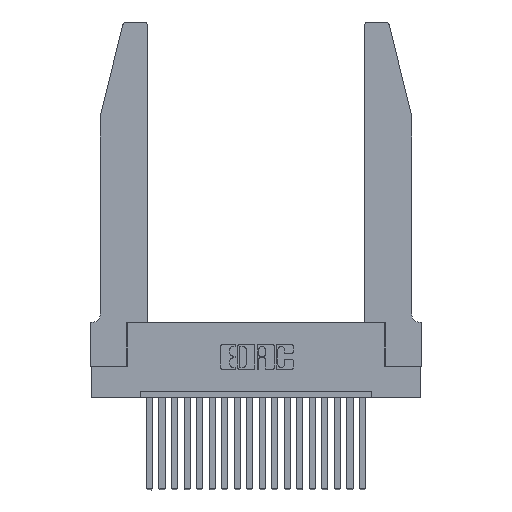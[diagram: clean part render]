
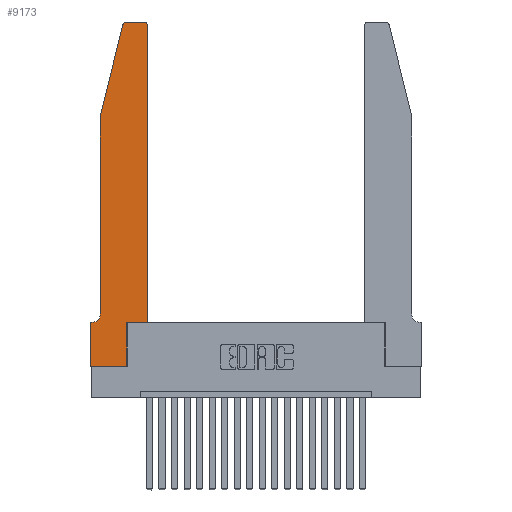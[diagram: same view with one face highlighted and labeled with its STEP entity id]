
A CAD part, top view. The second image highlights one B-rep face of the part: STEP entity #9173.
In plain terms, the highlighted planar face has unit normal (0, 0, 1).
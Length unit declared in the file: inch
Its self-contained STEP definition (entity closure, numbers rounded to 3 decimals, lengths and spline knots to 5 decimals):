
#276 = VERTEX_POINT ( 'NONE', #17920 ) ;
#367 = EDGE_CURVE ( 'NONE', #18900, #5737, #6683, .T. ) ;
#470 = CARTESIAN_POINT ( 'NONE',  ( 0., 0.35, 0.37 ) ) ;
#474 = CARTESIAN_POINT ( 'NONE',  ( 0.0755, 2., 0.37 ) ) ;
#629 = ORIENTED_EDGE ( 'NONE', *, *, #16393, .T. ) ;
#804 = CARTESIAN_POINT ( 'NONE',  ( 0.284, 2.72, 0.37 ) ) ;
#1341 = CARTESIAN_POINT ( 'NONE',  ( 0., 0.35, 0.37 ) ) ;
#1422 = VERTEX_POINT ( 'NONE', #15681 ) ;
#1963 = DIRECTION ( 'NONE',  ( 0., 1., 0. ) ) ;
#1997 = VERTEX_POINT ( 'NONE', #16521 ) ;
#2380 = ORIENTED_EDGE ( 'NONE', *, *, #7766, .T. ) ;
#2518 = DIRECTION ( 'NONE',  ( 1., 0., 0. ) ) ;
#2613 = LINE ( 'NONE', #474, #13183 ) ;
#2767 = VECTOR ( 'NONE', #1963, 39.37008 ) ;
#3095 = LINE ( 'NONE', #8594, #20072 ) ;
#3139 = CARTESIAN_POINT ( 'NONE',  ( 0.2865, 0., 0.37 ) ) ;
#3298 = ORIENTED_EDGE ( 'NONE', *, *, #17960, .T. ) ;
#3741 = CARTESIAN_POINT ( 'NONE',  ( 0.4205, 2.75, 0.37 ) ) ;
#3867 = VECTOR ( 'NONE', #13098, 39.37008 ) ;
#4355 = VERTEX_POINT ( 'NONE', #9360 ) ;
#4455 = VERTEX_POINT ( 'NONE', #3139 ) ;
#4566 = CARTESIAN_POINT ( 'NONE',  ( 0.0755, 2., 0.37 ) ) ;
#4745 = CARTESIAN_POINT ( 'NONE',  ( 0.25487, 2.72718, 0.37 ) ) ;
#4773 = VECTOR ( 'NONE', #19649, 39.37008 ) ;
#4788 = AXIS2_PLACEMENT_3D ( 'NONE', #14901, #16583, #8051 ) ;
#5555 = ORIENTED_EDGE ( 'NONE', *, *, #17258, .T. ) ;
#5737 = VERTEX_POINT ( 'NONE', #470 ) ;
#6047 = ORIENTED_EDGE ( 'NONE', *, *, #11536, .T. ) ;
#6191 = VECTOR ( 'NONE', #14361, 39.37008 ) ;
#6246 = DIRECTION ( 'NONE',  ( 0., 0., 1. ) ) ;
#6342 = CARTESIAN_POINT ( 'NONE',  ( 0.4505, 0.35, 0.37 ) ) ;
#6538 = DIRECTION ( 'NONE',  ( 1., 0., 0. ) ) ;
#6541 = VERTEX_POINT ( 'NONE', #4745 ) ;
#6654 = CARTESIAN_POINT ( 'NONE',  ( 0.2865, 0.35, 0.37 ) ) ;
#6683 = LINE ( 'NONE', #15209, #6191 ) ;
#6728 = CARTESIAN_POINT ( 'NONE',  ( 0.4505, 0.35, 0.37 ) ) ;
#7055 = DIRECTION ( 'NONE',  ( -1., 0., 0. ) ) ;
#7310 = ORIENTED_EDGE ( 'NONE', *, *, #21116, .T. ) ;
#7766 = EDGE_CURVE ( 'NONE', #19684, #18900, #10150, .T. ) ;
#7827 = PLANE ( 'NONE',  #13759 ) ;
#7865 = CARTESIAN_POINT ( 'NONE',  ( 0.4505, 2.72, 0.37 ) ) ;
#8051 = DIRECTION ( 'NONE',  ( 1., 0., 0. ) ) ;
#8155 = LINE ( 'NONE', #6342, #4773 ) ;
#8370 = CIRCLE ( 'NONE', #4788, 0.03 ) ;
#8379 = ORIENTED_EDGE ( 'NONE', *, *, #8538, .T. ) ;
#8538 = EDGE_CURVE ( 'NONE', #5737, #1997, #10610, .T. ) ;
#8594 = CARTESIAN_POINT ( 'NONE',  ( 0.2605, 2.75, 0.37 ) ) ;
#8809 = VECTOR ( 'NONE', #17312, 39.37008 ) ;
#9173 = ADVANCED_FACE ( 'NONE', ( #19567 ), #7827, .T. ) ;
#9360 = CARTESIAN_POINT ( 'NONE',  ( 0.4505, 0.35, 0.37 ) ) ;
#10059 = AXIS2_PLACEMENT_3D ( 'NONE', #804, #12324, #2518 ) ;
#10150 = CIRCLE ( 'NONE', #18430, 0.07 ) ;
#10610 = LINE ( 'NONE', #10720, #8809 ) ;
#10720 = CARTESIAN_POINT ( 'NONE',  ( 0., 0., 0.37 ) ) ;
#10819 = EDGE_CURVE ( 'NONE', #4455, #20757, #11882, .T. ) ;
#11406 = CARTESIAN_POINT ( 'NONE',  ( 0., 0., 0.37 ) ) ;
#11536 = EDGE_CURVE ( 'NONE', #13530, #1422, #3095, .T. ) ;
#11608 = ORIENTED_EDGE ( 'NONE', *, *, #367, .T. ) ;
#11882 = LINE ( 'NONE', #6654, #3867 ) ;
#12091 = CARTESIAN_POINT ( 'NONE',  ( 0.2865, 0.35, 0.37 ) ) ;
#12164 = LINE ( 'NONE', #4566, #18604 ) ;
#12324 = DIRECTION ( 'NONE',  ( 0., 0., 1. ) ) ;
#12583 = DIRECTION ( 'NONE',  ( -0.239, -0.971, 0. ) ) ;
#12602 = ORIENTED_EDGE ( 'NONE', *, *, #18326, .T. ) ;
#13098 = DIRECTION ( 'NONE',  ( 0., 1., 0. ) ) ;
#13183 = VECTOR ( 'NONE', #12583, 39.37008 ) ;
#13507 = ORIENTED_EDGE ( 'NONE', *, *, #20832, .T. ) ;
#13530 = VERTEX_POINT ( 'NONE', #3741 ) ;
#13759 = AXIS2_PLACEMENT_3D ( 'NONE', #1341, #6246, #19400 ) ;
#13806 = EDGE_LOOP ( 'NONE', ( #6047, #3298, #13507, #629, #2380, #11608, #8379, #12602, #14019, #13824, #5555, #7310 ) ) ;
#13824 = ORIENTED_EDGE ( 'NONE', *, *, #18267, .T. ) ;
#14019 = ORIENTED_EDGE ( 'NONE', *, *, #10819, .T. ) ;
#14361 = DIRECTION ( 'NONE',  ( -1., 0., 0. ) ) ;
#14372 = CARTESIAN_POINT ( 'NONE',  ( 0.0055, 0.35, 0.37 ) ) ;
#14901 = CARTESIAN_POINT ( 'NONE',  ( 0.4205, 2.72, 0.37 ) ) ;
#15209 = CARTESIAN_POINT ( 'NONE',  ( 0.0755, 0.35, 0.37 ) ) ;
#15681 = CARTESIAN_POINT ( 'NONE',  ( 0.284, 2.75, 0.37 ) ) ;
#16393 = EDGE_CURVE ( 'NONE', #276, #19684, #12164, .T. ) ;
#16521 = CARTESIAN_POINT ( 'NONE',  ( 0., 0., 0.37 ) ) ;
#16583 = DIRECTION ( 'NONE',  ( 0., 0., 1. ) ) ;
#16988 = DIRECTION ( 'NONE',  ( -1., 0., 0. ) ) ;
#17209 = LINE ( 'NONE', #6728, #2767 ) ;
#17258 = EDGE_CURVE ( 'NONE', #4355, #18194, #17209, .T. ) ;
#17312 = DIRECTION ( 'NONE',  ( 0., -1., 0. ) ) ;
#17692 = CIRCLE ( 'NONE', #10059, 0.03 ) ;
#17920 = CARTESIAN_POINT ( 'NONE',  ( 0.0755, 2., 0.37 ) ) ;
#17960 = EDGE_CURVE ( 'NONE', #1422, #6541, #17692, .T. ) ;
#18194 = VERTEX_POINT ( 'NONE', #7865 ) ;
#18267 = EDGE_CURVE ( 'NONE', #20757, #4355, #8155, .T. ) ;
#18326 = EDGE_CURVE ( 'NONE', #1997, #4455, #18704, .T. ) ;
#18347 = DIRECTION ( 'NONE',  ( 0., 0., -1. ) ) ;
#18430 = AXIS2_PLACEMENT_3D ( 'NONE', #18498, #18347, #7055 ) ;
#18498 = CARTESIAN_POINT ( 'NONE',  ( 0.0055, 0.42, 0.37 ) ) ;
#18604 = VECTOR ( 'NONE', #21272, 39.37008 ) ;
#18704 = LINE ( 'NONE', #11406, #19721 ) ;
#18900 = VERTEX_POINT ( 'NONE', #14372 ) ;
#19400 = DIRECTION ( 'NONE',  ( 1., 0., 0. ) ) ;
#19567 = FACE_OUTER_BOUND ( 'NONE', #13806, .T. ) ;
#19649 = DIRECTION ( 'NONE',  ( 1., 0., 0. ) ) ;
#19684 = VERTEX_POINT ( 'NONE', #20106 ) ;
#19721 = VECTOR ( 'NONE', #6538, 39.37008 ) ;
#20072 = VECTOR ( 'NONE', #16988, 39.37008 ) ;
#20106 = CARTESIAN_POINT ( 'NONE',  ( 0.0755, 0.42, 0.37 ) ) ;
#20757 = VERTEX_POINT ( 'NONE', #12091 ) ;
#20832 = EDGE_CURVE ( 'NONE', #6541, #276, #2613, .T. ) ;
#21116 = EDGE_CURVE ( 'NONE', #18194, #13530, #8370, .T. ) ;
#21272 = DIRECTION ( 'NONE',  ( 0., -1., 0. ) ) ;
